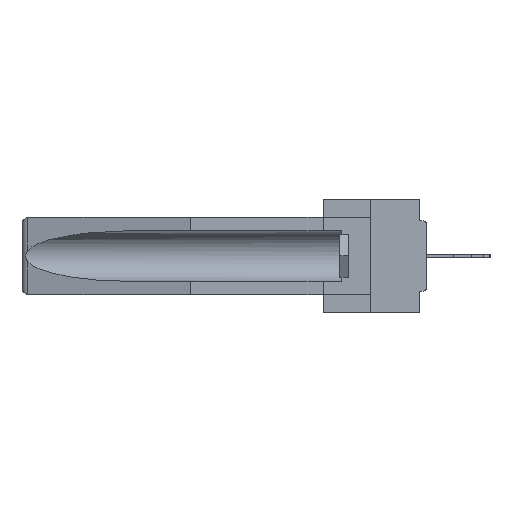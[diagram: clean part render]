
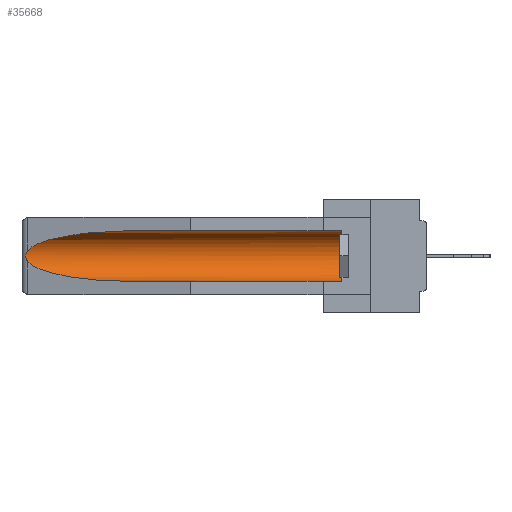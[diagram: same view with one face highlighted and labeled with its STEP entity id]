
A CAD part, left-side view. The second image highlights one B-rep face of the part: STEP entity #35668.
In plain terms, the highlighted cylindrical face has radius 2.857 mm (diameter 5.715 mm), a partial arc.
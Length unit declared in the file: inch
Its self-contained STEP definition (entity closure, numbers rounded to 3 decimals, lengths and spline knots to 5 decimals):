
#20 = EDGE_CURVE ( 'NONE', #13959, #10072, #37602, .T. ) ;
#620 = CARTESIAN_POINT ( 'NONE',  ( 0.155, -0.30754, -0.1715 ) ) ;
#1024 = DIRECTION ( 'NONE',  ( 0., 1., 0. ) ) ;
#1310 = DIRECTION ( 'NONE',  ( 0., -1., 0. ) ) ;
#2385 = ORIENTED_EDGE ( 'NONE', *, *, #4513, .T. ) ;
#2935 = CARTESIAN_POINT ( 'NONE',  ( 0.26537, 1.52718, -0.14972 ) ) ;
#3277 = CARTESIAN_POINT ( 'NONE',  ( 0.155, 1.07973, -0.284 ) ) ;
#3364 = CARTESIAN_POINT ( 'NONE',  ( 0.2675, 1.53308, -0.16763 ) ) ;
#3568 = CARTESIAN_POINT ( 'NONE',  ( 0.26597, 1.52961, -0.15275 ) ) ;
#4289 = CARTESIAN_POINT ( 'NONE',  ( 0.26537, 1.52718, -0.19328 ) ) ;
#4513 = EDGE_CURVE ( 'NONE', #40470, #13959, #5335, .T. ) ;
#5263 = CARTESIAN_POINT ( 'NONE',  ( 0.26537, 1.52718, -0.14972 ) ) ;
#5335 = CIRCLE ( 'NONE', #13257, 0.1125 ) ;
#6469 = CARTESIAN_POINT ( 'NONE',  ( 0.155, 0.126, -0.284 ) ) ;
#8138 = VECTOR ( 'NONE', #33283, 39.37008 ) ;
#8942 = EDGE_CURVE ( 'NONE', #40470, #18206, #14201, .T. ) ;
#9188 = AXIS2_PLACEMENT_3D ( 'NONE', #620, #1024, #13240 ) ;
#9330 = CARTESIAN_POINT ( 'NONE',  ( 0.26655, 1.53094, -0.18657 ) ) ;
#9746 = CARTESIAN_POINT ( 'NONE',  ( 0.26654, 1.53092, -0.15636 ) ) ;
#9908 = CARTESIAN_POINT ( 'NONE',  ( 0.155, 0.126, -0.059 ) ) ;
#10004 = CARTESIAN_POINT ( 'NONE',  ( 0.155, 0.126, -0.1715 ) ) ;
#10072 = VERTEX_POINT ( 'NONE', #16150 ) ;
#10816 = DIRECTION ( 'NONE',  ( 0., 0., 1. ) ) ;
#13240 = DIRECTION ( 'NONE',  ( 0., 0., 1. ) ) ;
#13257 = AXIS2_PLACEMENT_3D ( 'NONE', #10004, #1310, #10816 ) ;
#13949 = ORIENTED_EDGE ( 'NONE', *, *, #23532, .T. ) ;
#13959 = VERTEX_POINT ( 'NONE', #9908 ) ;
#14201 = LINE ( 'NONE', #20426, #8138 ) ;
#15330 = CARTESIAN_POINT ( 'NONE',  ( 0.26537, 1.52718, -0.19328 ) ) ;
#16148 = CARTESIAN_POINT ( 'NONE',  ( 0.2673, 1.53269, -0.17917 ) ) ;
#16150 = CARTESIAN_POINT ( 'NONE',  ( 0.155, 1.07973, -0.059 ) ) ;
#16965 = CYLINDRICAL_SURFACE ( 'NONE', #9188, 0.1125 ) ;
#18058 = CARTESIAN_POINT ( 'NONE',  ( 0.21114, 1.30732, -0.059 ) ) ;
#18206 = VERTEX_POINT ( 'NONE', #26894 ) ;
#18559 = CARTESIAN_POINT ( 'NONE',  ( 0.26537, 1.52718, -0.19328 ) ) ;
#19047 = CARTESIAN_POINT ( 'NONE',  ( 0.26597, 1.5296, -0.19026 ) ) ;
#19366 = CARTESIAN_POINT ( 'NONE',  ( 0.21114, 1.30732, -0.284 ) ) ;
#20426 = CARTESIAN_POINT ( 'NONE',  ( 0.155, -0.30754, -0.284 ) ) ;
#20967 = CARTESIAN_POINT ( 'NONE',  ( 0.155, 1.07973, -0.059 ) ) ;
#20975 =( BOUNDED_CURVE ( )  B_SPLINE_CURVE ( 3, ( #20967, #18058, #33637, #5263 ),
 .UNSPECIFIED., .F., .F. ) 
 B_SPLINE_CURVE_WITH_KNOTS ( ( 4, 4 ),
 ( 4.71239, 6.08839 ),
 .UNSPECIFIED. ) 
 CURVE ( )  GEOMETRIC_REPRESENTATION_ITEM ( )  RATIONAL_B_SPLINE_CURVE ( ( 1., 0.848, 0.848, 1. ) ) 
 REPRESENTATION_ITEM ( '' )  );
#21410 = DIRECTION ( 'NONE',  ( 0., 1., 0. ) ) ;
#23532 = EDGE_CURVE ( 'NONE', #30269, #18206, #29700, .T. ) ;
#25067 = CARTESIAN_POINT ( 'NONE',  ( 0.2673, 1.5327, -0.16383 ) ) ;
#26088 = EDGE_CURVE ( 'NONE', #26241, #30269, #32013, .T. ) ;
#26241 = VERTEX_POINT ( 'NONE', #39170 ) ;
#26723 = ORIENTED_EDGE ( 'NONE', *, *, #33294, .T. ) ;
#26894 = CARTESIAN_POINT ( 'NONE',  ( 0.155, 1.07973, -0.284 ) ) ;
#28728 = ORIENTED_EDGE ( 'NONE', *, *, #20, .T. ) ;
#29700 =( BOUNDED_CURVE ( )  B_SPLINE_CURVE ( 3, ( #18559, #31830, #19366, #3277 ),
 .UNSPECIFIED., .F., .F. ) 
 B_SPLINE_CURVE_WITH_KNOTS ( ( 4, 4 ),
 ( 0.1948, 1.5708 ),
 .UNSPECIFIED. ) 
 CURVE ( )  GEOMETRIC_REPRESENTATION_ITEM ( )  RATIONAL_B_SPLINE_CURVE ( ( 1., 0.848, 0.848, 1. ) ) 
 REPRESENTATION_ITEM ( '' )  );
#30269 = VERTEX_POINT ( 'NONE', #4289 ) ;
#30659 = VECTOR ( 'NONE', #21410, 39.37008 ) ;
#31830 = CARTESIAN_POINT ( 'NONE',  ( 0.25451, 1.48313, -0.24835 ) ) ;
#31913 = CARTESIAN_POINT ( 'NONE',  ( 0.2675, 1.53308, -0.17534 ) ) ;
#32013 = B_SPLINE_CURVE_WITH_KNOTS ( 'NONE', 3,
 ( #2935, #3568, #9746, #25067, #3364, #31913, #16148, #9330, #19047, #15330 ),
 .UNSPECIFIED., .F., .F.,
 ( 4, 2, 2, 2, 4 ),
 ( 0., 0.00029, 0.00058, 0.00087, 0.00117 ),
 .UNSPECIFIED. ) ;
#33283 = DIRECTION ( 'NONE',  ( 0., 1., 0. ) ) ;
#33294 = EDGE_CURVE ( 'NONE', #10072, #26241, #20975, .T. ) ;
#33637 = CARTESIAN_POINT ( 'NONE',  ( 0.25451, 1.48313, -0.09465 ) ) ;
#34505 = CARTESIAN_POINT ( 'NONE',  ( 0.155, -0.30754, -0.059 ) ) ;
#35668 = ADVANCED_FACE ( 'NONE', ( #39154 ), #16965, .F. ) ;
#37430 = ORIENTED_EDGE ( 'NONE', *, *, #26088, .T. ) ;
#37602 = LINE ( 'NONE', #34505, #30659 ) ;
#38659 = ORIENTED_EDGE ( 'NONE', *, *, #8942, .F. ) ;
#39154 = FACE_OUTER_BOUND ( 'NONE', #39767, .T. ) ;
#39170 = CARTESIAN_POINT ( 'NONE',  ( 0.26537, 1.52718, -0.14972 ) ) ;
#39767 = EDGE_LOOP ( 'NONE', ( #26723, #37430, #13949, #38659, #2385, #28728 ) ) ;
#40470 = VERTEX_POINT ( 'NONE', #6469 ) ;
